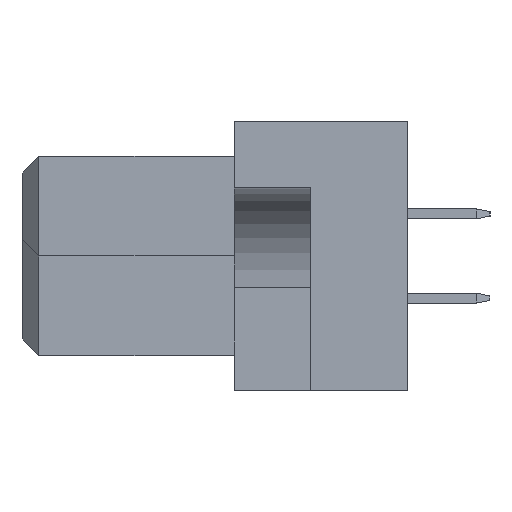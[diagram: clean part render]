
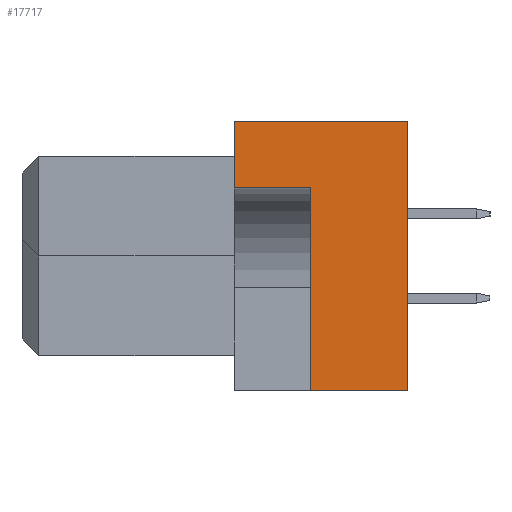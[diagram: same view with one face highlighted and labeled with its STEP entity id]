
A CAD part, left-side view. The second image highlights one B-rep face of the part: STEP entity #17717.
In plain terms, the highlighted planar face has unit normal (-1, 0, 0).
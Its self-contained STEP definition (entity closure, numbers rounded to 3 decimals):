
#144 = AXIS2_PLACEMENT_3D ( 'NONE', #12025, #24636, #9780 ) ;
#223 = DIRECTION ( 'NONE',  ( 0., 0., 1. ) ) ;
#884 = VECTOR ( 'NONE', #25511, 1000. ) ;
#1245 = VECTOR ( 'NONE', #223, 1000. ) ;
#1584 = VERTEX_POINT ( 'NONE', #24140 ) ;
#1823 = LINE ( 'NONE', #21161, #884 ) ;
#2013 = VECTOR ( 'NONE', #7643, 1000. ) ;
#2423 = ORIENTED_EDGE ( 'NONE', *, *, #27005, .F. ) ;
#2798 = VERTEX_POINT ( 'NONE', #10420 ) ;
#3434 = LINE ( 'NONE', #9739, #2013 ) ;
#4387 = VECTOR ( 'NONE', #6826, 1000. ) ;
#4404 = VERTEX_POINT ( 'NONE', #22455 ) ;
#4541 = LINE ( 'NONE', #21904, #15005 ) ;
#5207 = CARTESIAN_POINT ( 'NONE',  ( -47.5, 0., -4.05 ) ) ;
#5275 = LINE ( 'NONE', #7368, #25401 ) ;
#6826 = DIRECTION ( 'NONE',  ( 0., -1., 0. ) ) ;
#6976 = ORIENTED_EDGE ( 'NONE', *, *, #7273, .F. ) ;
#7273 = EDGE_CURVE ( 'NONE', #1584, #4404, #1823, .T. ) ;
#7368 = CARTESIAN_POINT ( 'NONE',  ( -47.5, 0., 4.05 ) ) ;
#7643 = DIRECTION ( 'NONE',  ( 0., -1., 0. ) ) ;
#8936 = CARTESIAN_POINT ( 'NONE',  ( -47.5, 5.2, 4.05 ) ) ;
#9076 = CARTESIAN_POINT ( 'NONE',  ( -47.5, 0., 4.05 ) ) ;
#9153 = VERTEX_POINT ( 'NONE', #9076 ) ;
#9485 = EDGE_CURVE ( 'NONE', #4404, #23462, #4541, .T. ) ;
#9739 = CARTESIAN_POINT ( 'NONE',  ( -47.5, 5.2, -4.05 ) ) ;
#9780 = DIRECTION ( 'NONE',  ( 0., 0., -1. ) ) ;
#10420 = CARTESIAN_POINT ( 'NONE',  ( -47.5, 5.2, 4.05 ) ) ;
#11750 = EDGE_CURVE ( 'NONE', #2798, #9153, #21263, .T. ) ;
#12025 = CARTESIAN_POINT ( 'NONE',  ( -47.5, 5.2, 4.05 ) ) ;
#12770 = VERTEX_POINT ( 'NONE', #5207 ) ;
#12834 = ORIENTED_EDGE ( 'NONE', *, *, #11750, .F. ) ;
#13137 = LINE ( 'NONE', #8936, #1245 ) ;
#15005 = VECTOR ( 'NONE', #17699, 1000. ) ;
#16447 = EDGE_CURVE ( 'NONE', #1584, #12770, #3434, .T. ) ;
#17425 = EDGE_LOOP ( 'NONE', ( #2423, #18865, #6976, #21967, #19360, #12834 ) ) ;
#17699 = DIRECTION ( 'NONE',  ( 0., 1., 0. ) ) ;
#17717 = ADVANCED_FACE ( 'NONE', ( #22807 ), #26594, .F. ) ;
#18013 = DIRECTION ( 'NONE',  ( 0., 0., 1. ) ) ;
#18865 = ORIENTED_EDGE ( 'NONE', *, *, #9485, .F. ) ;
#19172 = CARTESIAN_POINT ( 'NONE',  ( -47.5, 5.2, 4.05 ) ) ;
#19360 = ORIENTED_EDGE ( 'NONE', *, *, #21826, .T. ) ;
#21161 = CARTESIAN_POINT ( 'NONE',  ( -47.5, 2.9, 2.05 ) ) ;
#21263 = LINE ( 'NONE', #19172, #4387 ) ;
#21826 = EDGE_CURVE ( 'NONE', #12770, #9153, #5275, .T. ) ;
#21904 = CARTESIAN_POINT ( 'NONE',  ( -47.5, 2.9, 2.05 ) ) ;
#21967 = ORIENTED_EDGE ( 'NONE', *, *, #16447, .T. ) ;
#22455 = CARTESIAN_POINT ( 'NONE',  ( -47.5, 2.9, 2.05 ) ) ;
#22807 = FACE_OUTER_BOUND ( 'NONE', #17425, .T. ) ;
#22874 = CARTESIAN_POINT ( 'NONE',  ( -47.5, 5.2, 2.05 ) ) ;
#23462 = VERTEX_POINT ( 'NONE', #22874 ) ;
#24140 = CARTESIAN_POINT ( 'NONE',  ( -47.5, 2.9, -4.05 ) ) ;
#24636 = DIRECTION ( 'NONE',  ( 1., 0., 0. ) ) ;
#25401 = VECTOR ( 'NONE', #18013, 1000. ) ;
#25511 = DIRECTION ( 'NONE',  ( 0., 0., 1. ) ) ;
#26594 = PLANE ( 'NONE',  #144 ) ;
#27005 = EDGE_CURVE ( 'NONE', #23462, #2798, #13137, .T. ) ;
